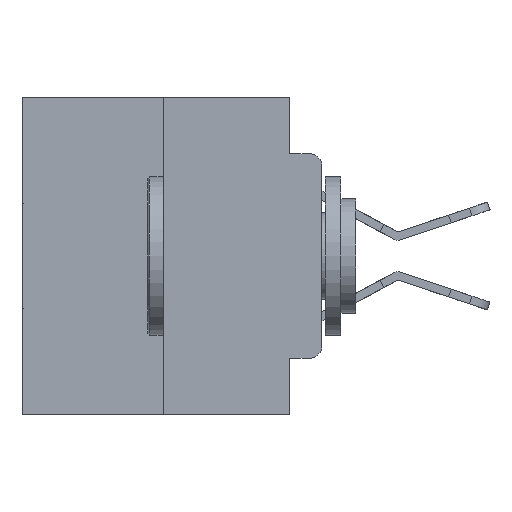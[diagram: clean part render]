
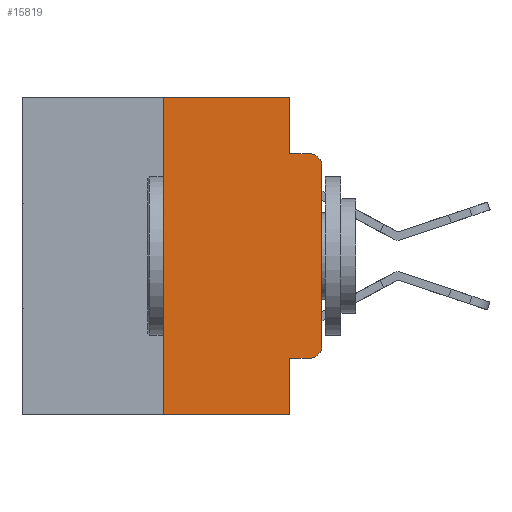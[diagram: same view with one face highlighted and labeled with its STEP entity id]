
A CAD part, left-side view. The second image highlights one B-rep face of the part: STEP entity #15819.
In plain terms, the highlighted planar face has unit normal (-1, 0, 0).
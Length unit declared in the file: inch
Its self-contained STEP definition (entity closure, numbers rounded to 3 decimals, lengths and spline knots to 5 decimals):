
#479 = ORIENTED_EDGE ( 'NONE', *, *, #30112, .T. ) ;
#824 = VERTEX_POINT ( 'NONE', #6290 ) ;
#1390 = DIRECTION ( 'NONE',  ( 0., 0., -1. ) ) ;
#1408 = AXIS2_PLACEMENT_3D ( 'NONE', #11474, #27431, #13838 ) ;
#2160 = LINE ( 'NONE', #10014, #14043 ) ;
#2826 = ORIENTED_EDGE ( 'NONE', *, *, #29901, .F. ) ;
#3026 = EDGE_CURVE ( 'NONE', #29773, #26817, #12408, .T. ) ;
#4019 = VECTOR ( 'NONE', #13322, 39.37008 ) ;
#4492 = VECTOR ( 'NONE', #29880, 39.37008 ) ;
#4701 = DIRECTION ( 'NONE',  ( -1., 0., 0. ) ) ;
#5011 = VECTOR ( 'NONE', #29201, 39.37008 ) ;
#5400 = VECTOR ( 'NONE', #29011, 39.37008 ) ;
#5599 = VERTEX_POINT ( 'NONE', #12682 ) ;
#6003 = VERTEX_POINT ( 'NONE', #9389 ) ;
#6103 = LINE ( 'NONE', #29905, #23828 ) ;
#6290 = CARTESIAN_POINT ( 'NONE',  ( 0., 0.051, 0. ) ) ;
#6680 = DIRECTION ( 'NONE',  ( 0., -1., 0. ) ) ;
#6888 = VERTEX_POINT ( 'NONE', #13020 ) ;
#7056 = VERTEX_POINT ( 'NONE', #20372 ) ;
#7821 = CIRCLE ( 'NONE', #19816, 0.02 ) ;
#7849 = EDGE_CURVE ( 'NONE', #824, #17941, #28989, .T. ) ;
#7981 = VERTEX_POINT ( 'NONE', #23563 ) ;
#8405 = ORIENTED_EDGE ( 'NONE', *, *, #26311, .T. ) ;
#8417 = EDGE_CURVE ( 'NONE', #7981, #7056, #7821, .T. ) ;
#9389 = CARTESIAN_POINT ( 'NONE',  ( 0., 0., -0.1085 ) ) ;
#10014 = CARTESIAN_POINT ( 'NONE',  ( 0., 0., 0. ) ) ;
#10313 = LINE ( 'NONE', #22404, #4019 ) ;
#11474 = CARTESIAN_POINT ( 'NONE',  ( 0., 0.02, -0.1085 ) ) ;
#12377 = DIRECTION ( 'NONE',  ( 0., 0., 1. ) ) ;
#12408 = LINE ( 'NONE', #21296, #5400 ) ;
#12552 = EDGE_CURVE ( 'NONE', #17941, #19996, #25904, .T. ) ;
#12682 = CARTESIAN_POINT ( 'NONE',  ( 0., 0.051, -0.5 ) ) ;
#13020 = CARTESIAN_POINT ( 'NONE',  ( 0., 0.051, -0.4115 ) ) ;
#13322 = DIRECTION ( 'NONE',  ( 0., -1., 0. ) ) ;
#13838 = DIRECTION ( 'NONE',  ( 0., 0., -1. ) ) ;
#13918 = FACE_OUTER_BOUND ( 'NONE', #23073, .T. ) ;
#14030 = DIRECTION ( 'NONE',  ( 0., -1., 0. ) ) ;
#14043 = VECTOR ( 'NONE', #12377, 39.37008 ) ;
#14380 = CIRCLE ( 'NONE', #1408, 0.02 ) ;
#14686 = EDGE_CURVE ( 'NONE', #6888, #7981, #10313, .T. ) ;
#14953 = VECTOR ( 'NONE', #6680, 39.37008 ) ;
#15588 = DIRECTION ( 'NONE',  ( 1., 0., 0. ) ) ;
#15819 = ADVANCED_FACE ( 'NONE', ( #13918 ), #28971, .F. ) ;
#15865 = CARTESIAN_POINT ( 'NONE',  ( 0., 0.051, -0.0885 ) ) ;
#15875 = CARTESIAN_POINT ( 'NONE',  ( 0., 0.02, -0.0885 ) ) ;
#16043 = ORIENTED_EDGE ( 'NONE', *, *, #18649, .T. ) ;
#16778 = ORIENTED_EDGE ( 'NONE', *, *, #8417, .T. ) ;
#17663 = VECTOR ( 'NONE', #25950, 39.37008 ) ;
#17767 = CARTESIAN_POINT ( 'NONE',  ( 0., 0.051, 0. ) ) ;
#17941 = VERTEX_POINT ( 'NONE', #15865 ) ;
#18264 = AXIS2_PLACEMENT_3D ( 'NONE', #29156, #15588, #1390 ) ;
#18592 = CARTESIAN_POINT ( 'NONE',  ( 0., 0.02, -0.3915 ) ) ;
#18649 = EDGE_CURVE ( 'NONE', #6003, #19996, #14380, .T. ) ;
#19816 = AXIS2_PLACEMENT_3D ( 'NONE', #18592, #4701, #20895 ) ;
#19996 = VERTEX_POINT ( 'NONE', #15875 ) ;
#20256 = LINE ( 'NONE', #20502, #14953 ) ;
#20372 = CARTESIAN_POINT ( 'NONE',  ( 0., 0., -0.3915 ) ) ;
#20502 = CARTESIAN_POINT ( 'NONE',  ( 0., 0.473, 0. ) ) ;
#20895 = DIRECTION ( 'NONE',  ( 0., 0., -1. ) ) ;
#21007 = CARTESIAN_POINT ( 'NONE',  ( 0., 0.25, 0. ) ) ;
#21296 = CARTESIAN_POINT ( 'NONE',  ( 0., 0.25, 0. ) ) ;
#22404 = CARTESIAN_POINT ( 'NONE',  ( 0., 0.051, -0.4115 ) ) ;
#23073 = EDGE_LOOP ( 'NONE', ( #8405, #16043, #23552, #24249, #27056, #29917, #479, #2826, #27436, #16778 ) ) ;
#23552 = ORIENTED_EDGE ( 'NONE', *, *, #12552, .F. ) ;
#23563 = CARTESIAN_POINT ( 'NONE',  ( 0., 0.02, -0.4115 ) ) ;
#23679 = CARTESIAN_POINT ( 'NONE',  ( 0., 0.051, -0.0885 ) ) ;
#23828 = VECTOR ( 'NONE', #14030, 39.37008 ) ;
#24249 = ORIENTED_EDGE ( 'NONE', *, *, #7849, .F. ) ;
#25904 = LINE ( 'NONE', #23679, #17663 ) ;
#25950 = DIRECTION ( 'NONE',  ( 0., -1., 0. ) ) ;
#26311 = EDGE_CURVE ( 'NONE', #7056, #6003, #2160, .T. ) ;
#26817 = VERTEX_POINT ( 'NONE', #21007 ) ;
#27056 = ORIENTED_EDGE ( 'NONE', *, *, #29352, .F. ) ;
#27431 = DIRECTION ( 'NONE',  ( -1., 0., 0. ) ) ;
#27436 = ORIENTED_EDGE ( 'NONE', *, *, #14686, .T. ) ;
#27603 = CARTESIAN_POINT ( 'NONE',  ( 0., 0.051, 0. ) ) ;
#27729 = CARTESIAN_POINT ( 'NONE',  ( 0., 0.25, -0.5 ) ) ;
#28971 = PLANE ( 'NONE',  #18264 ) ;
#28989 = LINE ( 'NONE', #27603, #4492 ) ;
#29011 = DIRECTION ( 'NONE',  ( 0., 0., 1. ) ) ;
#29156 = CARTESIAN_POINT ( 'NONE',  ( 0., 0.473, 0. ) ) ;
#29201 = DIRECTION ( 'NONE',  ( 0., 0., -1. ) ) ;
#29352 = EDGE_CURVE ( 'NONE', #26817, #824, #20256, .T. ) ;
#29466 = LINE ( 'NONE', #17767, #5011 ) ;
#29773 = VERTEX_POINT ( 'NONE', #27729 ) ;
#29880 = DIRECTION ( 'NONE',  ( 0., 0., -1. ) ) ;
#29901 = EDGE_CURVE ( 'NONE', #6888, #5599, #29466, .T. ) ;
#29905 = CARTESIAN_POINT ( 'NONE',  ( 0., 0.473, -0.5 ) ) ;
#29917 = ORIENTED_EDGE ( 'NONE', *, *, #3026, .F. ) ;
#30112 = EDGE_CURVE ( 'NONE', #29773, #5599, #6103, .T. ) ;
